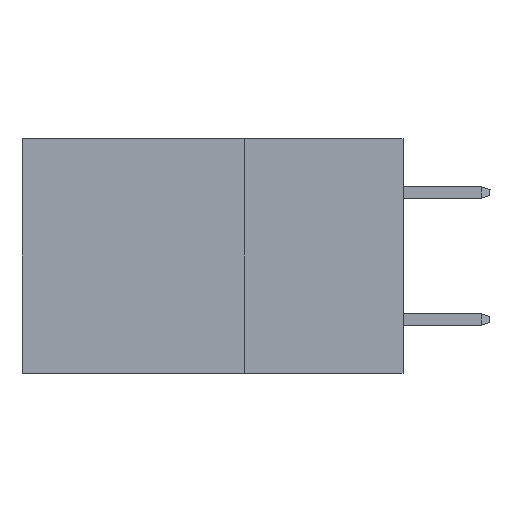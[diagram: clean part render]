
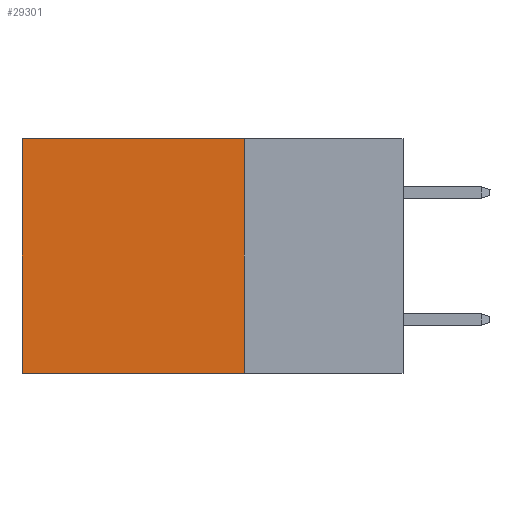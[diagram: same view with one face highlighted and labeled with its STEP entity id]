
A CAD part, left-side view. The second image highlights one B-rep face of the part: STEP entity #29301.
In plain terms, the highlighted planar face has unit normal (-1, 0, 0).
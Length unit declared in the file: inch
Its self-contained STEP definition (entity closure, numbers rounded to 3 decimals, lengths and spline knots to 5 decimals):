
#1179 = CARTESIAN_POINT ( 'NONE',  ( 0.2875, 0.6, -0.37 ) ) ;
#4430 = PLANE ( 'NONE',  #32835 ) ;
#5224 = CARTESIAN_POINT ( 'NONE',  ( 0.2875, 0.25, 0. ) ) ;
#6653 = DIRECTION ( 'NONE',  ( 0., 1., 0. ) ) ;
#7881 = EDGE_CURVE ( 'NONE', #13465, #20220, #11928, .T. ) ;
#8458 = EDGE_CURVE ( 'NONE', #25644, #33315, #24482, .T. ) ;
#9218 = CARTESIAN_POINT ( 'NONE',  ( 0.2875, 0.6, 0. ) ) ;
#10367 = ORIENTED_EDGE ( 'NONE', *, *, #8458, .F. ) ;
#10420 = DIRECTION ( 'NONE',  ( 0., 1., 0. ) ) ;
#11536 = CARTESIAN_POINT ( 'NONE',  ( 0.2875, 0.25, 0. ) ) ;
#11846 = EDGE_LOOP ( 'NONE', ( #12131, #26106, #10367, #33500 ) ) ;
#11928 = LINE ( 'NONE', #9218, #28050 ) ;
#12131 = ORIENTED_EDGE ( 'NONE', *, *, #7881, .T. ) ;
#13465 = VERTEX_POINT ( 'NONE', #18555 ) ;
#14965 = LINE ( 'NONE', #22820, #19803 ) ;
#18555 = CARTESIAN_POINT ( 'NONE',  ( 0.2875, 0.6, 0. ) ) ;
#19384 = VECTOR ( 'NONE', #22101, 39.37008 ) ;
#19803 = VECTOR ( 'NONE', #6653, 39.37008 ) ;
#20220 = VERTEX_POINT ( 'NONE', #1179 ) ;
#22101 = DIRECTION ( 'NONE',  ( 0., 0., -1. ) ) ;
#22820 = CARTESIAN_POINT ( 'NONE',  ( 0.2875, 0.25, -0.37 ) ) ;
#22972 = DIRECTION ( 'NONE',  ( 1., 0., 0. ) ) ;
#23550 = EDGE_CURVE ( 'NONE', #25644, #13465, #23887, .T. ) ;
#23887 = LINE ( 'NONE', #26426, #26593 ) ;
#24482 = LINE ( 'NONE', #11536, #19384 ) ;
#25179 = FACE_OUTER_BOUND ( 'NONE', #11846, .T. ) ;
#25366 = DIRECTION ( 'NONE',  ( 0., 0., -1. ) ) ;
#25644 = VERTEX_POINT ( 'NONE', #5224 ) ;
#26106 = ORIENTED_EDGE ( 'NONE', *, *, #29391, .F. ) ;
#26426 = CARTESIAN_POINT ( 'NONE',  ( 0.2875, 0.25, 0. ) ) ;
#26593 = VECTOR ( 'NONE', #10420, 39.37008 ) ;
#27400 = DIRECTION ( 'NONE',  ( 0., 0., -1. ) ) ;
#28050 = VECTOR ( 'NONE', #27400, 39.37008 ) ;
#29301 = ADVANCED_FACE ( 'NONE', ( #25179 ), #4430, .F. ) ;
#29391 = EDGE_CURVE ( 'NONE', #33315, #20220, #14965, .T. ) ;
#30606 = CARTESIAN_POINT ( 'NONE',  ( 0.2875, 0.25, 0. ) ) ;
#30860 = CARTESIAN_POINT ( 'NONE',  ( 0.2875, 0.25, -0.37 ) ) ;
#32835 = AXIS2_PLACEMENT_3D ( 'NONE', #30606, #22972, #25366 ) ;
#33315 = VERTEX_POINT ( 'NONE', #30860 ) ;
#33500 = ORIENTED_EDGE ( 'NONE', *, *, #23550, .T. ) ;
